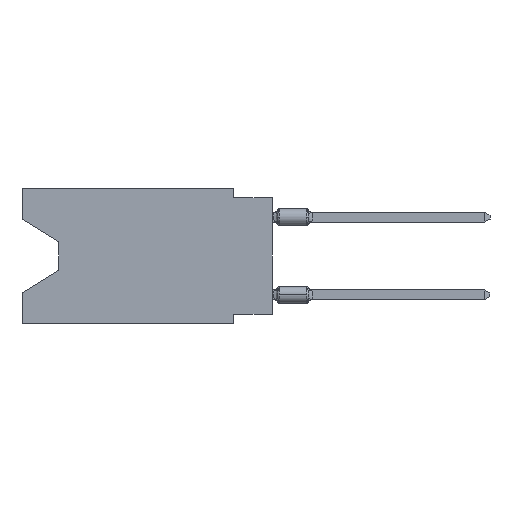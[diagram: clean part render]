
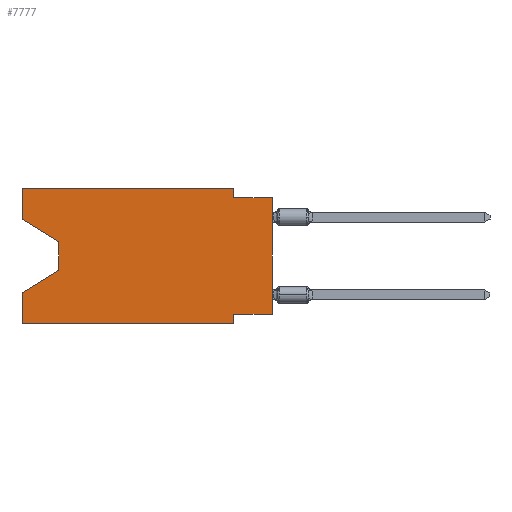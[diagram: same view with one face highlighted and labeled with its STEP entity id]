
A CAD part, left-side view. The second image highlights one B-rep face of the part: STEP entity #7777.
In plain terms, the highlighted planar face has unit normal (-1, 0, 0).
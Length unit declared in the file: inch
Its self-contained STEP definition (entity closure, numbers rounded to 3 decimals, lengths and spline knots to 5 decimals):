
#215 = ORIENTED_EDGE ( 'NONE', *, *, #16065, .T. ) ;
#495 = DIRECTION ( 'NONE',  ( 0., -1., 0. ) ) ;
#783 = ORIENTED_EDGE ( 'NONE', *, *, #7279, .T. ) ;
#837 = AXIS2_PLACEMENT_3D ( 'NONE', #12809, #24672, #18909 ) ;
#1265 = CARTESIAN_POINT ( 'NONE',  ( 0., 0.1, 0. ) ) ;
#2016 = VECTOR ( 'NONE', #495, 39.37008 ) ;
#2864 = CARTESIAN_POINT ( 'NONE',  ( 0., 0., -0.325 ) ) ;
#3645 = CARTESIAN_POINT ( 'NONE',  ( 0., 0.645, 0. ) ) ;
#3807 = VECTOR ( 'NONE', #18759, 39.37008 ) ;
#3822 = VECTOR ( 'NONE', #15110, 39.37008 ) ;
#4214 = VECTOR ( 'NONE', #19308, 39.37008 ) ;
#4686 = CARTESIAN_POINT ( 'NONE',  ( 0., 0.645, -0.08025 ) ) ;
#4859 = ORIENTED_EDGE ( 'NONE', *, *, #6287, .F. ) ;
#4908 = LINE ( 'NONE', #23374, #3822 ) ;
#5095 = VECTOR ( 'NONE', #10995, 39.37008 ) ;
#5172 = ORIENTED_EDGE ( 'NONE', *, *, #12665, .F. ) ;
#5457 = EDGE_CURVE ( 'NONE', #7034, #6856, #8717, .T. ) ;
#5878 = CARTESIAN_POINT ( 'NONE',  ( 0., 0., -0.325 ) ) ;
#6050 = EDGE_LOOP ( 'NONE', ( #215, #783, #18930, #9649, #22943, #5172, #23775, #23002, #25096, #11128, #23771, #4859 ) ) ;
#6058 = EDGE_CURVE ( 'NONE', #21734, #20327, #14820, .T. ) ;
#6287 = EDGE_CURVE ( 'NONE', #6846, #21734, #20263, .T. ) ;
#6327 = CARTESIAN_POINT ( 'NONE',  ( 0., 0.55, -0.212 ) ) ;
#6846 = VERTEX_POINT ( 'NONE', #4686 ) ;
#6856 = VERTEX_POINT ( 'NONE', #22880 ) ;
#7034 = VERTEX_POINT ( 'NONE', #5878 ) ;
#7279 = EDGE_CURVE ( 'NONE', #12071, #19434, #11258, .T. ) ;
#7389 = DIRECTION ( 'NONE',  ( 0., 0., 1. ) ) ;
#7394 = EDGE_CURVE ( 'NONE', #19434, #21071, #21083, .T. ) ;
#7454 = VERTEX_POINT ( 'NONE', #9416 ) ;
#7777 = ADVANCED_FACE ( 'NONE', ( #25038 ), #16546, .F. ) ;
#8717 = LINE ( 'NONE', #2864, #15361 ) ;
#8827 = LINE ( 'NONE', #1265, #4214 ) ;
#9227 = CARTESIAN_POINT ( 'NONE',  ( 0., 0., -0.025 ) ) ;
#9416 = CARTESIAN_POINT ( 'NONE',  ( 0., 0.1, -0.025 ) ) ;
#9649 = ORIENTED_EDGE ( 'NONE', *, *, #22794, .F. ) ;
#9785 = DIRECTION ( 'NONE',  ( 0., 0., 1. ) ) ;
#10392 = CARTESIAN_POINT ( 'NONE',  ( 0., 0.55, -0.138 ) ) ;
#10624 = VERTEX_POINT ( 'NONE', #17904 ) ;
#10995 = DIRECTION ( 'NONE',  ( 0., -1., 0. ) ) ;
#11128 = ORIENTED_EDGE ( 'NONE', *, *, #22815, .F. ) ;
#11258 = LINE ( 'NONE', #18841, #11858 ) ;
#11343 = CARTESIAN_POINT ( 'NONE',  ( 0., 0.645, -0.35 ) ) ;
#11396 = LINE ( 'NONE', #19499, #5095 ) ;
#11646 = LINE ( 'NONE', #13911, #13455 ) ;
#11858 = VECTOR ( 'NONE', #13263, 39.37008 ) ;
#12071 = VERTEX_POINT ( 'NONE', #10392 ) ;
#12665 = EDGE_CURVE ( 'NONE', #6856, #10624, #11646, .T. ) ;
#12809 = CARTESIAN_POINT ( 'NONE',  ( 0., 0.645, 0. ) ) ;
#13070 = VECTOR ( 'NONE', #13176, 39.37008 ) ;
#13176 = DIRECTION ( 'NONE',  ( 0., -1., 0. ) ) ;
#13263 = DIRECTION ( 'NONE',  ( 0., 0., -1. ) ) ;
#13455 = VECTOR ( 'NONE', #17491, 39.37008 ) ;
#13911 = CARTESIAN_POINT ( 'NONE',  ( 0., 0.1, -0.35 ) ) ;
#14046 = EDGE_CURVE ( 'NONE', #14827, #10624, #15030, .T. ) ;
#14768 = VERTEX_POINT ( 'NONE', #9227 ) ;
#14820 = LINE ( 'NONE', #18682, #2016 ) ;
#14827 = VERTEX_POINT ( 'NONE', #11343 ) ;
#15030 = LINE ( 'NONE', #21412, #13070 ) ;
#15110 = DIRECTION ( 'NONE',  ( 0., -0.855, -0.519 ) ) ;
#15279 = CARTESIAN_POINT ( 'NONE',  ( 0., 0., 0. ) ) ;
#15361 = VECTOR ( 'NONE', #22689, 39.37008 ) ;
#16065 = EDGE_CURVE ( 'NONE', #6846, #12071, #4908, .T. ) ;
#16098 = EDGE_CURVE ( 'NONE', #7454, #14768, #11396, .T. ) ;
#16546 = PLANE ( 'NONE',  #837 ) ;
#17240 = DIRECTION ( 'NONE',  ( 0., 0.855, -0.519 ) ) ;
#17348 = VECTOR ( 'NONE', #7389, 39.37008 ) ;
#17491 = DIRECTION ( 'NONE',  ( 0., 0., -1. ) ) ;
#17904 = CARTESIAN_POINT ( 'NONE',  ( 0., 0.1, -0.35 ) ) ;
#18682 = CARTESIAN_POINT ( 'NONE',  ( 0., 0.645, 0. ) ) ;
#18759 = DIRECTION ( 'NONE',  ( 0., 0., 1. ) ) ;
#18841 = CARTESIAN_POINT ( 'NONE',  ( 0., 0.55, -0.138 ) ) ;
#18909 = DIRECTION ( 'NONE',  ( 0., 0., -1. ) ) ;
#18930 = ORIENTED_EDGE ( 'NONE', *, *, #7394, .T. ) ;
#19229 = CARTESIAN_POINT ( 'NONE',  ( 0., 0.55, -0.212 ) ) ;
#19308 = DIRECTION ( 'NONE',  ( 0., 0., -1. ) ) ;
#19434 = VERTEX_POINT ( 'NONE', #6327 ) ;
#19499 = CARTESIAN_POINT ( 'NONE',  ( 0., 0., -0.025 ) ) ;
#20256 = VECTOR ( 'NONE', #9785, 39.37008 ) ;
#20263 = LINE ( 'NONE', #22139, #20256 ) ;
#20327 = VERTEX_POINT ( 'NONE', #24134 ) ;
#20727 = CARTESIAN_POINT ( 'NONE',  ( 0., 0.645, -0.26975 ) ) ;
#20997 = LINE ( 'NONE', #15279, #3807 ) ;
#21071 = VERTEX_POINT ( 'NONE', #20727 ) ;
#21083 = LINE ( 'NONE', #19229, #25873 ) ;
#21167 = LINE ( 'NONE', #23449, #17348 ) ;
#21412 = CARTESIAN_POINT ( 'NONE',  ( 0., 0.645, -0.35 ) ) ;
#21734 = VERTEX_POINT ( 'NONE', #3645 ) ;
#22006 = EDGE_CURVE ( 'NONE', #7034, #14768, #20997, .T. ) ;
#22139 = CARTESIAN_POINT ( 'NONE',  ( 0., 0.645, 0. ) ) ;
#22689 = DIRECTION ( 'NONE',  ( 0., 1., 0. ) ) ;
#22794 = EDGE_CURVE ( 'NONE', #14827, #21071, #21167, .T. ) ;
#22815 = EDGE_CURVE ( 'NONE', #20327, #7454, #8827, .T. ) ;
#22880 = CARTESIAN_POINT ( 'NONE',  ( 0., 0.1, -0.325 ) ) ;
#22943 = ORIENTED_EDGE ( 'NONE', *, *, #14046, .T. ) ;
#23002 = ORIENTED_EDGE ( 'NONE', *, *, #22006, .T. ) ;
#23374 = CARTESIAN_POINT ( 'NONE',  ( 0., 0.645, -0.08025 ) ) ;
#23449 = CARTESIAN_POINT ( 'NONE',  ( 0., 0.645, 0. ) ) ;
#23771 = ORIENTED_EDGE ( 'NONE', *, *, #6058, .F. ) ;
#23775 = ORIENTED_EDGE ( 'NONE', *, *, #5457, .F. ) ;
#24134 = CARTESIAN_POINT ( 'NONE',  ( 0., 0.1, 0. ) ) ;
#24672 = DIRECTION ( 'NONE',  ( 1., 0., 0. ) ) ;
#25038 = FACE_OUTER_BOUND ( 'NONE', #6050, .T. ) ;
#25096 = ORIENTED_EDGE ( 'NONE', *, *, #16098, .F. ) ;
#25873 = VECTOR ( 'NONE', #17240, 39.37008 ) ;
